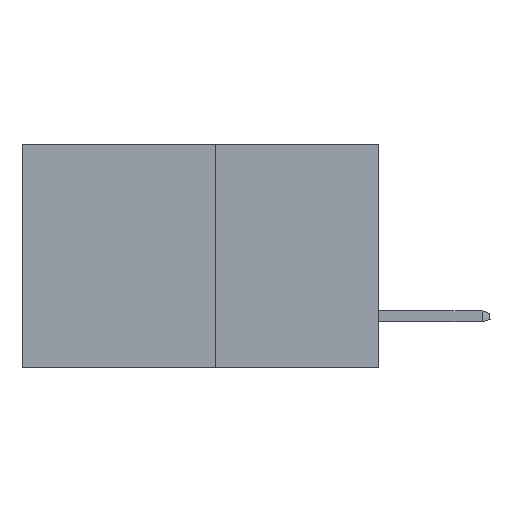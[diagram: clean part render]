
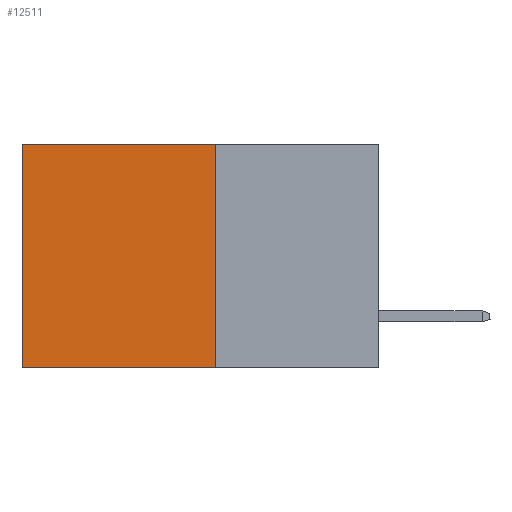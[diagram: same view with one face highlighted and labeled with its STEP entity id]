
A CAD part, left-side view. The second image highlights one B-rep face of the part: STEP entity #12511.
In plain terms, the highlighted planar face has unit normal (-1, 0, 0).
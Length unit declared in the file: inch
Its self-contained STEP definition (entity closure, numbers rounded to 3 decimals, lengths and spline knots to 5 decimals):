
#403 = DIRECTION ( 'NONE',  ( 0., 0., -1. ) ) ;
#1996 = VERTEX_POINT ( 'NONE', #9834 ) ;
#2364 = LINE ( 'NONE', #11244, #13117 ) ;
#2770 = CARTESIAN_POINT ( 'NONE',  ( 0.277, 0.27, -0.37 ) ) ;
#3679 = EDGE_CURVE ( 'NONE', #13033, #1996, #6346, .T. ) ;
#3846 = VECTOR ( 'NONE', #14625, 39.37008 ) ;
#4225 = DIRECTION ( 'NONE',  ( 0., 1., 0. ) ) ;
#4699 = ORIENTED_EDGE ( 'NONE', *, *, #3679, .T. ) ;
#4894 = AXIS2_PLACEMENT_3D ( 'NONE', #6194, #17256, #8939 ) ;
#5067 = VECTOR ( 'NONE', #4225, 39.37008 ) ;
#6126 = PLANE ( 'NONE',  #4894 ) ;
#6194 = CARTESIAN_POINT ( 'NONE',  ( 0.277, 0.27, -0.37 ) ) ;
#6346 = LINE ( 'NONE', #11146, #16940 ) ;
#6790 = ORIENTED_EDGE ( 'NONE', *, *, #14414, .F. ) ;
#7187 = DIRECTION ( 'NONE',  ( 0., 0., -1. ) ) ;
#7579 = CARTESIAN_POINT ( 'NONE',  ( 0.277, 0.59, 0. ) ) ;
#8287 = EDGE_CURVE ( 'NONE', #11551, #12775, #2364, .T. ) ;
#8939 = DIRECTION ( 'NONE',  ( 0., 0., -1. ) ) ;
#9065 = CARTESIAN_POINT ( 'NONE',  ( 0.277, 0.27, 0. ) ) ;
#9460 = CARTESIAN_POINT ( 'NONE',  ( 0.277, 0.27, -0.37 ) ) ;
#9477 = FACE_OUTER_BOUND ( 'NONE', #15813, .T. ) ;
#9674 = CARTESIAN_POINT ( 'NONE',  ( 0.277, 0.27, 0. ) ) ;
#9720 = ORIENTED_EDGE ( 'NONE', *, *, #8287, .F. ) ;
#9834 = CARTESIAN_POINT ( 'NONE',  ( 0.277, 0.59, -0.37 ) ) ;
#10469 = EDGE_CURVE ( 'NONE', #11551, #13033, #15433, .T. ) ;
#11146 = CARTESIAN_POINT ( 'NONE',  ( 0.277, 0.59, -0.37 ) ) ;
#11244 = CARTESIAN_POINT ( 'NONE',  ( 0.277, 0.27, -0.37 ) ) ;
#11351 = ORIENTED_EDGE ( 'NONE', *, *, #10469, .T. ) ;
#11551 = VERTEX_POINT ( 'NONE', #9674 ) ;
#12511 = ADVANCED_FACE ( 'NONE', ( #9477 ), #6126, .F. ) ;
#12775 = VERTEX_POINT ( 'NONE', #9460 ) ;
#13033 = VERTEX_POINT ( 'NONE', #7579 ) ;
#13117 = VECTOR ( 'NONE', #7187, 39.37008 ) ;
#14414 = EDGE_CURVE ( 'NONE', #12775, #1996, #16198, .T. ) ;
#14625 = DIRECTION ( 'NONE',  ( 0., 1., 0. ) ) ;
#15433 = LINE ( 'NONE', #9065, #3846 ) ;
#15813 = EDGE_LOOP ( 'NONE', ( #4699, #6790, #9720, #11351 ) ) ;
#16198 = LINE ( 'NONE', #2770, #5067 ) ;
#16940 = VECTOR ( 'NONE', #403, 39.37008 ) ;
#17256 = DIRECTION ( 'NONE',  ( 1., 0., 0. ) ) ;
